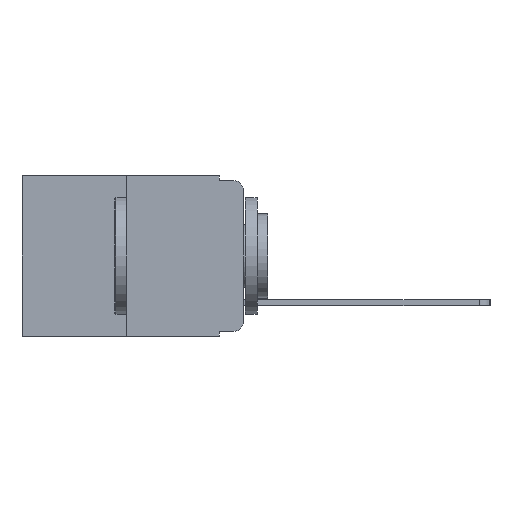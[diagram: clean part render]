
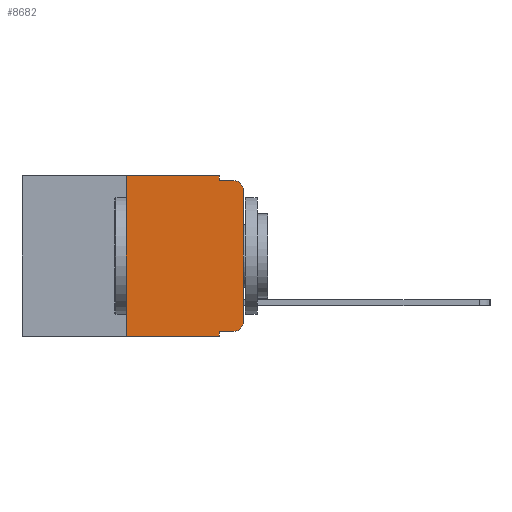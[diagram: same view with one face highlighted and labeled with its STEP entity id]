
A CAD part, left-side view. The second image highlights one B-rep face of the part: STEP entity #8682.
In plain terms, the highlighted planar face has unit normal (-1, 0, 0).
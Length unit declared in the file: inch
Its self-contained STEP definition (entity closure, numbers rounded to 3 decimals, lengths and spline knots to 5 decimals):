
#369 = VECTOR ( 'NONE', #7675, 39.37008 ) ;
#503 = DIRECTION ( 'NONE',  ( 0., -1., 0. ) ) ;
#718 = DIRECTION ( 'NONE',  ( 0., 0., -1. ) ) ;
#740 = LINE ( 'NONE', #11074, #369 ) ;
#956 = DIRECTION ( 'NONE',  ( 0., 0., 1. ) ) ;
#1121 = LINE ( 'NONE', #4010, #6969 ) ;
#1576 = VERTEX_POINT ( 'NONE', #10258 ) ;
#1648 = CARTESIAN_POINT ( 'NONE',  ( 0., 0.051, -0.01 ) ) ;
#1684 = ORIENTED_EDGE ( 'NONE', *, *, #10220, .F. ) ;
#1777 = LINE ( 'NONE', #6330, #4550 ) ;
#1783 = VERTEX_POINT ( 'NONE', #7236 ) ;
#1869 = ORIENTED_EDGE ( 'NONE', *, *, #10966, .F. ) ;
#1973 = AXIS2_PLACEMENT_3D ( 'NONE', #3570, #11614, #4765 ) ;
#2779 = CIRCLE ( 'NONE', #1973, 0.02 ) ;
#3046 = LINE ( 'NONE', #11124, #6170 ) ;
#3549 = VECTOR ( 'NONE', #956, 39.37008 ) ;
#3570 = CARTESIAN_POINT ( 'NONE',  ( 0., 0.02, -0.313 ) ) ;
#3612 = PLANE ( 'NONE',  #6683 ) ;
#3791 = CARTESIAN_POINT ( 'NONE',  ( 0., 0., -0.03 ) ) ;
#3896 = ORIENTED_EDGE ( 'NONE', *, *, #13218, .T. ) ;
#3904 = VERTEX_POINT ( 'NONE', #10342 ) ;
#4010 = CARTESIAN_POINT ( 'NONE',  ( 0., 0.051, -0.333 ) ) ;
#4271 = ORIENTED_EDGE ( 'NONE', *, *, #12489, .F. ) ;
#4550 = VECTOR ( 'NONE', #503, 39.37008 ) ;
#4593 = VECTOR ( 'NONE', #7732, 39.37008 ) ;
#4765 = DIRECTION ( 'NONE',  ( 0., 0., -1. ) ) ;
#4907 = LINE ( 'NONE', #14647, #13618 ) ;
#5568 = ORIENTED_EDGE ( 'NONE', *, *, #9424, .T. ) ;
#5801 = VECTOR ( 'NONE', #9012, 39.37008 ) ;
#5960 = DIRECTION ( 'NONE',  ( 1., 0., 0. ) ) ;
#6170 = VECTOR ( 'NONE', #13378, 39.37008 ) ;
#6330 = CARTESIAN_POINT ( 'NONE',  ( 0., 0.473, 0. ) ) ;
#6566 = EDGE_CURVE ( 'NONE', #13853, #7284, #740, .T. ) ;
#6683 = AXIS2_PLACEMENT_3D ( 'NONE', #10537, #5960, #13890 ) ;
#6751 = VERTEX_POINT ( 'NONE', #9123 ) ;
#6969 = VECTOR ( 'NONE', #7490, 39.37008 ) ;
#7236 = CARTESIAN_POINT ( 'NONE',  ( 0., 0.25, 0. ) ) ;
#7284 = VERTEX_POINT ( 'NONE', #11296 ) ;
#7342 = ORIENTED_EDGE ( 'NONE', *, *, #11726, .F. ) ;
#7490 = DIRECTION ( 'NONE',  ( 0., -1., 0. ) ) ;
#7635 = LINE ( 'NONE', #11126, #4593 ) ;
#7675 = DIRECTION ( 'NONE',  ( 0., -1., 0. ) ) ;
#7684 = DIRECTION ( 'NONE',  ( -1., 0., 0. ) ) ;
#7732 = DIRECTION ( 'NONE',  ( 0., 0., -1. ) ) ;
#7864 = CARTESIAN_POINT ( 'NONE',  ( 0., 0.051, -0.01 ) ) ;
#7910 = CARTESIAN_POINT ( 'NONE',  ( 0., 0., 0. ) ) ;
#8053 = ORIENTED_EDGE ( 'NONE', *, *, #6566, .T. ) ;
#8266 = CIRCLE ( 'NONE', #14200, 0.02 ) ;
#8284 = EDGE_CURVE ( 'NONE', #1783, #1576, #1777, .T. ) ;
#8372 = VERTEX_POINT ( 'NONE', #12208 ) ;
#8585 = ORIENTED_EDGE ( 'NONE', *, *, #8650, .T. ) ;
#8650 = EDGE_CURVE ( 'NONE', #3904, #6751, #2779, .T. ) ;
#8682 = ADVANCED_FACE ( 'NONE', ( #11626 ), #3612, .F. ) ;
#8909 = VERTEX_POINT ( 'NONE', #1648 ) ;
#9012 = DIRECTION ( 'NONE',  ( 0., -1., 0. ) ) ;
#9123 = CARTESIAN_POINT ( 'NONE',  ( 0., 0., -0.313 ) ) ;
#9424 = EDGE_CURVE ( 'NONE', #8372, #3904, #1121, .T. ) ;
#9687 = LINE ( 'NONE', #7910, #3549 ) ;
#9968 = VERTEX_POINT ( 'NONE', #3791 ) ;
#9975 = CARTESIAN_POINT ( 'NONE',  ( 0., 0.25, -0.343 ) ) ;
#10220 = EDGE_CURVE ( 'NONE', #8372, #7284, #7635, .T. ) ;
#10229 = DIRECTION ( 'NONE',  ( 0., 0., -1. ) ) ;
#10258 = CARTESIAN_POINT ( 'NONE',  ( 0., 0.051, 0. ) ) ;
#10342 = CARTESIAN_POINT ( 'NONE',  ( 0., 0.02, -0.333 ) ) ;
#10407 = ORIENTED_EDGE ( 'NONE', *, *, #8284, .F. ) ;
#10537 = CARTESIAN_POINT ( 'NONE',  ( 0., 0.473, 0. ) ) ;
#10966 = EDGE_CURVE ( 'NONE', #13853, #1783, #3046, .T. ) ;
#11074 = CARTESIAN_POINT ( 'NONE',  ( 0., 0.473, -0.343 ) ) ;
#11124 = CARTESIAN_POINT ( 'NONE',  ( 0., 0.25, 0. ) ) ;
#11126 = CARTESIAN_POINT ( 'NONE',  ( 0., 0.051, 0. ) ) ;
#11296 = CARTESIAN_POINT ( 'NONE',  ( 0., 0.051, -0.343 ) ) ;
#11614 = DIRECTION ( 'NONE',  ( -1., 0., 0. ) ) ;
#11626 = FACE_OUTER_BOUND ( 'NONE', #14350, .T. ) ;
#11726 = EDGE_CURVE ( 'NONE', #1576, #8909, #4907, .T. ) ;
#12208 = CARTESIAN_POINT ( 'NONE',  ( 0., 0.051, -0.333 ) ) ;
#12322 = ORIENTED_EDGE ( 'NONE', *, *, #13956, .T. ) ;
#12422 = CARTESIAN_POINT ( 'NONE',  ( 0., 0.02, -0.01 ) ) ;
#12489 = EDGE_CURVE ( 'NONE', #8909, #13313, #14808, .T. ) ;
#13218 = EDGE_CURVE ( 'NONE', #9968, #13313, #8266, .T. ) ;
#13313 = VERTEX_POINT ( 'NONE', #12422 ) ;
#13378 = DIRECTION ( 'NONE',  ( 0., 0., 1. ) ) ;
#13618 = VECTOR ( 'NONE', #10229, 39.37008 ) ;
#13853 = VERTEX_POINT ( 'NONE', #9975 ) ;
#13890 = DIRECTION ( 'NONE',  ( 0., 0., -1. ) ) ;
#13956 = EDGE_CURVE ( 'NONE', #6751, #9968, #9687, .T. ) ;
#14200 = AXIS2_PLACEMENT_3D ( 'NONE', #14433, #7684, #718 ) ;
#14350 = EDGE_LOOP ( 'NONE', ( #12322, #3896, #4271, #7342, #10407, #1869, #8053, #1684, #5568, #8585 ) ) ;
#14433 = CARTESIAN_POINT ( 'NONE',  ( 0., 0.02, -0.03 ) ) ;
#14647 = CARTESIAN_POINT ( 'NONE',  ( 0., 0.051, 0. ) ) ;
#14808 = LINE ( 'NONE', #7864, #5801 ) ;
